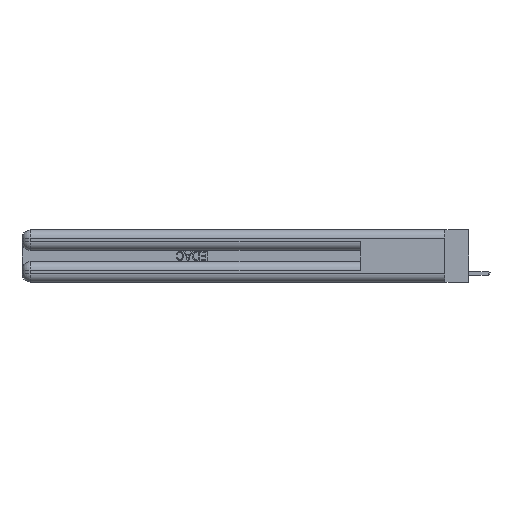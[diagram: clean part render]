
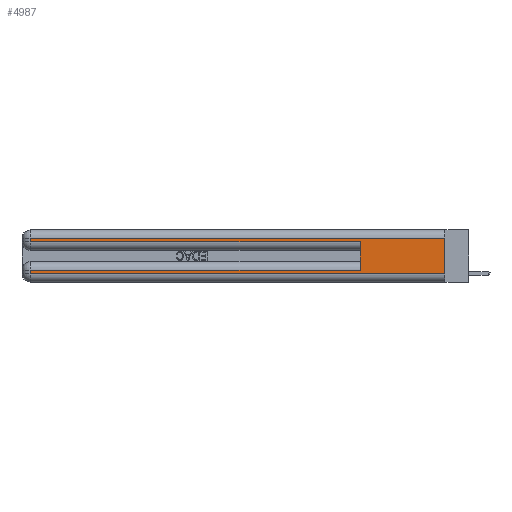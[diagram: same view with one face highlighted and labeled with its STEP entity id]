
A CAD part, left-side view. The second image highlights one B-rep face of the part: STEP entity #4987.
In plain terms, the highlighted planar face has unit normal (-1, 0, 0).
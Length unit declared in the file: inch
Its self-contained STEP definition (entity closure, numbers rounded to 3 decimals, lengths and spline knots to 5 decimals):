
#222 = DIRECTION ( 'NONE',  ( 1., 0., 0. ) ) ;
#311 = CARTESIAN_POINT ( 'NONE',  ( 0., 0., 0.06 ) ) ;
#353 = CARTESIAN_POINT ( 'NONE',  ( 0., 2.94, 0.37 ) ) ;
#555 = VECTOR ( 'NONE', #13080, 39.37008 ) ;
#836 = VECTOR ( 'NONE', #13251, 39.37008 ) ;
#1061 = DIRECTION ( 'NONE',  ( 0., 0., -1. ) ) ;
#1659 = CARTESIAN_POINT ( 'NONE',  ( 0., 2.94, 0.085 ) ) ;
#2349 = DIRECTION ( 'NONE',  ( 0., 0., -1. ) ) ;
#2526 = DIRECTION ( 'NONE',  ( 0., 0., -1. ) ) ;
#3098 = VERTEX_POINT ( 'NONE', #22171 ) ;
#3406 = VERTEX_POINT ( 'NONE', #8904 ) ;
#3437 = ORIENTED_EDGE ( 'NONE', *, *, #4412, .T. ) ;
#3766 = VECTOR ( 'NONE', #18883, 39.37008 ) ;
#3894 = VECTOR ( 'NONE', #12504, 39.37008 ) ;
#4005 = ORIENTED_EDGE ( 'NONE', *, *, #22101, .F. ) ;
#4013 = CARTESIAN_POINT ( 'NONE',  ( 0., 0., 0.06 ) ) ;
#4412 = EDGE_CURVE ( 'NONE', #21683, #13771, #9394, .T. ) ;
#4987 = ADVANCED_FACE ( 'NONE', ( #5439 ), #25396, .F. ) ;
#5413 = LINE ( 'NONE', #10547, #9646 ) ;
#5439 = FACE_OUTER_BOUND ( 'NONE', #26041, .T. ) ;
#6808 = CARTESIAN_POINT ( 'NONE',  ( 0., 0., 0.31 ) ) ;
#7129 = VECTOR ( 'NONE', #1061, 39.37008 ) ;
#7416 = VERTEX_POINT ( 'NONE', #1659 ) ;
#8904 = CARTESIAN_POINT ( 'NONE',  ( 0., 0.6, 0.085 ) ) ;
#9394 = LINE ( 'NONE', #4013, #17542 ) ;
#9646 = VECTOR ( 'NONE', #26767, 39.37008 ) ;
#10410 = CARTESIAN_POINT ( 'NONE',  ( 0., 0., 0.285 ) ) ;
#10547 = CARTESIAN_POINT ( 'NONE',  ( 0., 0., 0.085 ) ) ;
#10939 = EDGE_CURVE ( 'NONE', #13386, #13160, #25707, .T. ) ;
#12060 = EDGE_CURVE ( 'NONE', #3406, #7416, #5413, .T. ) ;
#12504 = DIRECTION ( 'NONE',  ( 0., -1., 0. ) ) ;
#13080 = DIRECTION ( 'NONE',  ( 0., 0., 1. ) ) ;
#13160 = VERTEX_POINT ( 'NONE', #14509 ) ;
#13251 = DIRECTION ( 'NONE',  ( 0., 1., 0. ) ) ;
#13386 = VERTEX_POINT ( 'NONE', #26148 ) ;
#13771 = VERTEX_POINT ( 'NONE', #311 ) ;
#14509 = CARTESIAN_POINT ( 'NONE',  ( 0., 2.94, 0.285 ) ) ;
#14545 = ORIENTED_EDGE ( 'NONE', *, *, #18500, .T. ) ;
#15002 = CARTESIAN_POINT ( 'NONE',  ( 0., 0., 0.37 ) ) ;
#15032 = AXIS2_PLACEMENT_3D ( 'NONE', #23397, #222, #2349 ) ;
#15082 = VECTOR ( 'NONE', #2526, 39.37008 ) ;
#15126 = ORIENTED_EDGE ( 'NONE', *, *, #12060, .T. ) ;
#15217 = ORIENTED_EDGE ( 'NONE', *, *, #10939, .T. ) ;
#15740 = LINE ( 'NONE', #15002, #15082 ) ;
#15970 = EDGE_CURVE ( 'NONE', #3098, #13771, #15740, .T. ) ;
#16161 = LINE ( 'NONE', #353, #3766 ) ;
#17542 = VECTOR ( 'NONE', #20867, 39.37008 ) ;
#18500 = EDGE_CURVE ( 'NONE', #13160, #24341, #20194, .T. ) ;
#18883 = DIRECTION ( 'NONE',  ( 0., 0., -1. ) ) ;
#19947 = EDGE_CURVE ( 'NONE', #3098, #13386, #21075, .T. ) ;
#20194 = LINE ( 'NONE', #10410, #3894 ) ;
#20455 = EDGE_CURVE ( 'NONE', #7416, #21683, #16161, .T. ) ;
#20867 = DIRECTION ( 'NONE',  ( 0., -1., 0. ) ) ;
#21075 = LINE ( 'NONE', #6808, #836 ) ;
#21190 = ORIENTED_EDGE ( 'NONE', *, *, #15970, .F. ) ;
#21321 = CARTESIAN_POINT ( 'NONE',  ( 0., 2.94, 0.37 ) ) ;
#21683 = VERTEX_POINT ( 'NONE', #22191 ) ;
#21984 = ORIENTED_EDGE ( 'NONE', *, *, #19947, .T. ) ;
#22101 = EDGE_CURVE ( 'NONE', #3406, #24341, #25639, .T. ) ;
#22171 = CARTESIAN_POINT ( 'NONE',  ( 0., 0., 0.31 ) ) ;
#22191 = CARTESIAN_POINT ( 'NONE',  ( 0., 2.94, 0.06 ) ) ;
#23397 = CARTESIAN_POINT ( 'NONE',  ( 0., 0., 0.37 ) ) ;
#24318 = CARTESIAN_POINT ( 'NONE',  ( 0., 0.6, 0.285 ) ) ;
#24341 = VERTEX_POINT ( 'NONE', #24318 ) ;
#25386 = CARTESIAN_POINT ( 'NONE',  ( 0., 0.6, 0.145 ) ) ;
#25396 = PLANE ( 'NONE',  #15032 ) ;
#25639 = LINE ( 'NONE', #25386, #555 ) ;
#25707 = LINE ( 'NONE', #21321, #7129 ) ;
#25998 = ORIENTED_EDGE ( 'NONE', *, *, #20455, .T. ) ;
#26041 = EDGE_LOOP ( 'NONE', ( #21190, #21984, #15217, #14545, #4005, #15126, #25998, #3437 ) ) ;
#26148 = CARTESIAN_POINT ( 'NONE',  ( 0., 2.94, 0.31 ) ) ;
#26767 = DIRECTION ( 'NONE',  ( 0., 1., 0. ) ) ;
